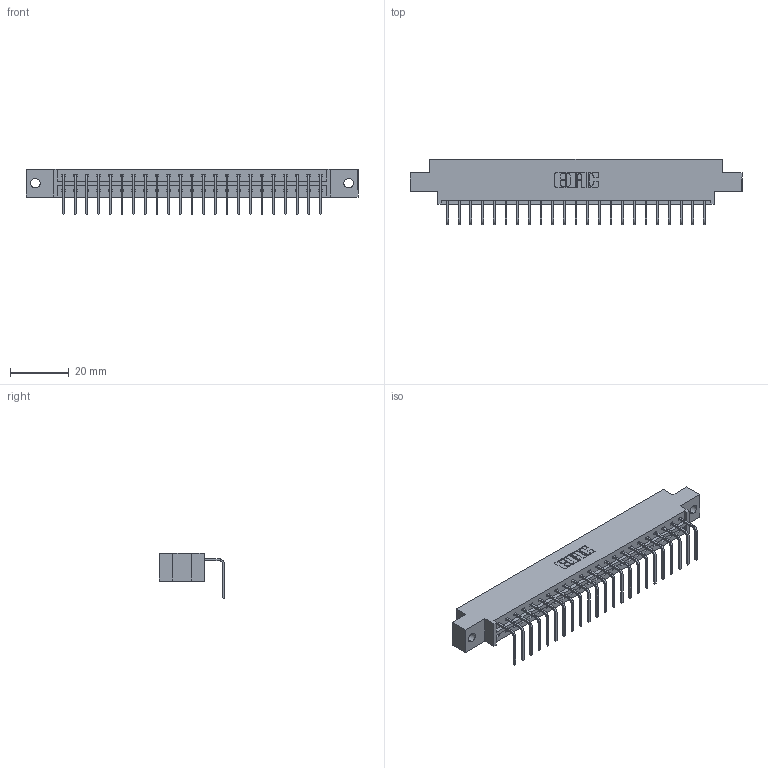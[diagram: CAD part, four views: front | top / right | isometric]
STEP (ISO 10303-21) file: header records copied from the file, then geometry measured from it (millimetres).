
FILE_DESCRIPTION (( 'STEP AP203' ), '1' );
FILE_NAME ('833-023-558-602.STEP', '2020-06-01T19:41:34', ( '' ), ( '' ), 'SwSTEP 2.0', 'SolidWorks 2020', '' );
FILE_SCHEMA (( 'CONFIG_CONTROL_DESIGN' ));
Length unit declared in the file: inch
Products named in the file (3): 345-292-001_558 Tail - 2; 833 Part_Offset - .128 Dia; 833-023-558-602
Assembly tree (24 placements, depth 2):
  833-023-558-602
    833 Part_Offset - .128 Dia
    345-292-001_558 Tail - 2  x23
Bounding box: 112.67 x 22.17 x 15.37 mm (x, y, z)
Volume: 10987 mm3; surface area: 12159 mm2
Topology: 24 solids, 24 shells, 1498 faces, 4509 edges, 2974 vertices
Faces by surface type: plane 1086, cylinder 412
Entity records: 16737 total; most frequent: CARTESIAN_POINT 2899, ORIENTED_EDGE 2858, DIRECTION 2483, EDGE_CURVE 1429, LINE 1301, VECTOR 1301, VERTEX_POINT 950, AXIS2_PLACEMENT_3D 591
